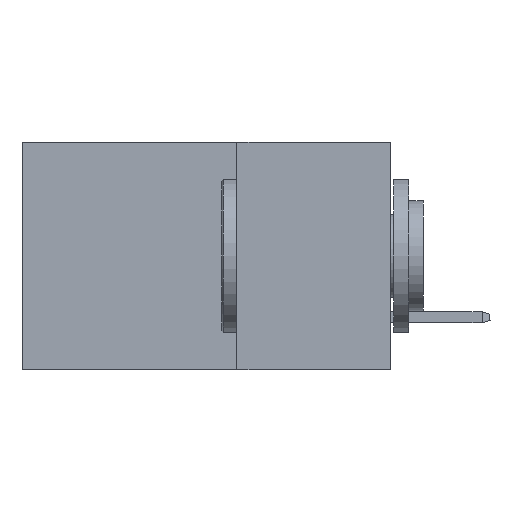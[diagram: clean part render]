
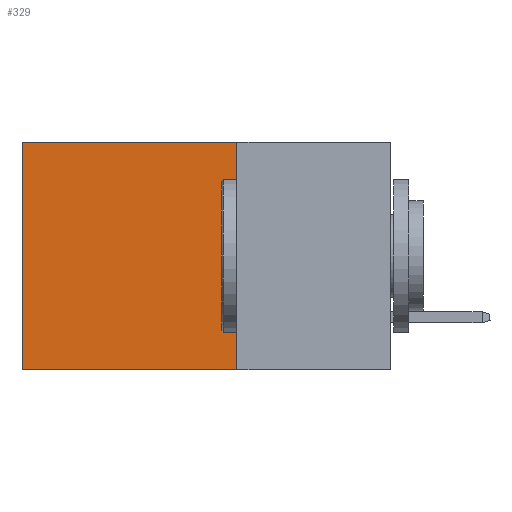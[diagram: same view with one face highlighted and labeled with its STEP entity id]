
A CAD part, left-side view. The second image highlights one B-rep face of the part: STEP entity #329.
In plain terms, the highlighted planar face has unit normal (-1, 0, 0).
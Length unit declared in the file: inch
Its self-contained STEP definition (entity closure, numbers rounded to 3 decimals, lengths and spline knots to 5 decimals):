
#329 = ADVANCED_FACE ( 'NONE', ( #12042 ), #14586, .F. ) ;
#580 = DIRECTION ( 'NONE',  ( 0., 1., 0. ) ) ;
#1239 = ORIENTED_EDGE ( 'NONE', *, *, #5476, .F. ) ;
#1448 = DIRECTION ( 'NONE',  ( 1., 0., 0. ) ) ;
#2873 = EDGE_CURVE ( 'NONE', #11721, #14254, #11953, .T. ) ;
#3035 = LINE ( 'NONE', #3186, #9876 ) ;
#3186 = CARTESIAN_POINT ( 'NONE',  ( 0.2875, 0.25, 0. ) ) ;
#3860 = EDGE_CURVE ( 'NONE', #11721, #5155, #3035, .T. ) ;
#4253 = CARTESIAN_POINT ( 'NONE',  ( 0.2875, 0.6, 0. ) ) ;
#5155 = VERTEX_POINT ( 'NONE', #8060 ) ;
#5476 = EDGE_CURVE ( 'NONE', #14254, #13263, #7734, .T. ) ;
#5551 = DIRECTION ( 'NONE',  ( 0., 1., 0. ) ) ;
#5995 = CARTESIAN_POINT ( 'NONE',  ( 0.2875, 0.6, -0.37 ) ) ;
#6292 = ORIENTED_EDGE ( 'NONE', *, *, #2873, .F. ) ;
#6306 = VECTOR ( 'NONE', #14261, 39.37008 ) ;
#6311 = CARTESIAN_POINT ( 'NONE',  ( 0.2875, 0.25, 0. ) ) ;
#7012 = EDGE_LOOP ( 'NONE', ( #9717, #1239, #6292, #14550 ) ) ;
#7734 = LINE ( 'NONE', #13850, #15087 ) ;
#8060 = CARTESIAN_POINT ( 'NONE',  ( 0.2875, 0.6, 0. ) ) ;
#8562 = DIRECTION ( 'NONE',  ( 0., 0., -1. ) ) ;
#8800 = CARTESIAN_POINT ( 'NONE',  ( 0.2875, 0.25, 0. ) ) ;
#9717 = ORIENTED_EDGE ( 'NONE', *, *, #11891, .T. ) ;
#9876 = VECTOR ( 'NONE', #5551, 39.37008 ) ;
#10201 = DIRECTION ( 'NONE',  ( 0., 0., -1. ) ) ;
#11167 = VECTOR ( 'NONE', #10201, 39.37008 ) ;
#11516 = AXIS2_PLACEMENT_3D ( 'NONE', #6311, #1448, #8562 ) ;
#11721 = VERTEX_POINT ( 'NONE', #8800 ) ;
#11891 = EDGE_CURVE ( 'NONE', #5155, #13263, #13418, .T. ) ;
#11953 = LINE ( 'NONE', #14240, #6306 ) ;
#12042 = FACE_OUTER_BOUND ( 'NONE', #7012, .T. ) ;
#13263 = VERTEX_POINT ( 'NONE', #5995 ) ;
#13418 = LINE ( 'NONE', #4253, #11167 ) ;
#13561 = CARTESIAN_POINT ( 'NONE',  ( 0.2875, 0.25, -0.37 ) ) ;
#13850 = CARTESIAN_POINT ( 'NONE',  ( 0.2875, 0.25, -0.37 ) ) ;
#14240 = CARTESIAN_POINT ( 'NONE',  ( 0.2875, 0.25, 0. ) ) ;
#14254 = VERTEX_POINT ( 'NONE', #13561 ) ;
#14261 = DIRECTION ( 'NONE',  ( 0., 0., -1. ) ) ;
#14550 = ORIENTED_EDGE ( 'NONE', *, *, #3860, .T. ) ;
#14586 = PLANE ( 'NONE',  #11516 ) ;
#15087 = VECTOR ( 'NONE', #580, 39.37008 ) ;
